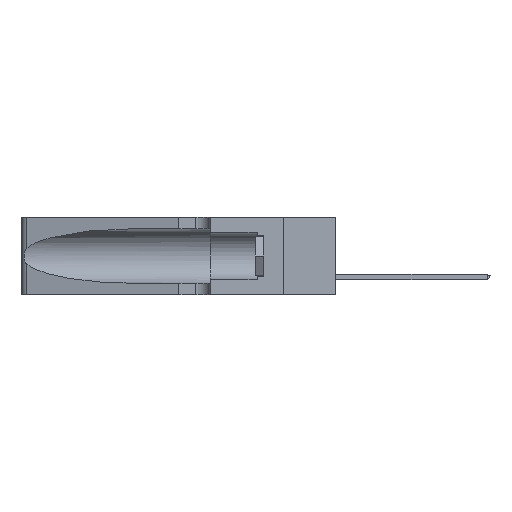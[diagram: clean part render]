
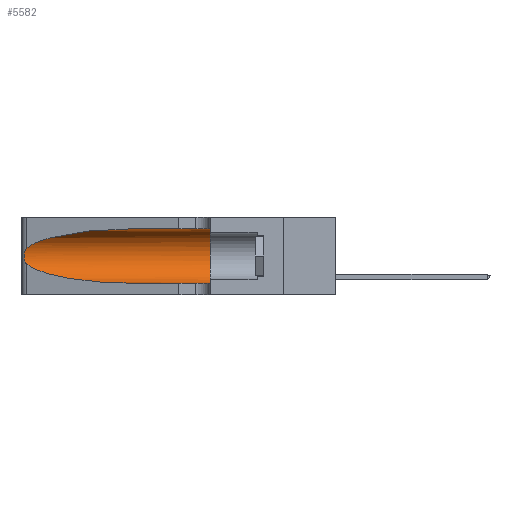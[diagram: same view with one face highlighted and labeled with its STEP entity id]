
A CAD part, left-side view. The second image highlights one B-rep face of the part: STEP entity #5582.
In plain terms, the highlighted cylindrical face has radius 3.308 mm (diameter 6.617 mm), a partial arc.
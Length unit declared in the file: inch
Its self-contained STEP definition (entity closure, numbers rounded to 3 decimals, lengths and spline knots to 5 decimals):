
#102 = CARTESIAN_POINT ( 'NONE',  ( 0.18966, 0.96281, 0.05475 ) ) ;
#1041 = CARTESIAN_POINT ( 'NONE',  ( 0.25787, 1.23484, 0.2124 ) ) ;
#1892 = CARTESIAN_POINT ( 'NONE',  ( 0.25555, 1.22994, 0.2215 ) ) ;
#1995 = CARTESIAN_POINT ( 'NONE',  ( 0.25856, 1.23593, 0.16098 ) ) ;
#2781 = DIRECTION ( 'NONE',  ( 0., -1., 0. ) ) ;
#3120 = CARTESIAN_POINT ( 'NONE',  ( 0.25487, 1.22718, 0.14631 ) ) ;
#3766 = CARTESIAN_POINT ( 'NONE',  ( 0.1305, 0.72297, 0.31525 ) ) ;
#3886 = CARTESIAN_POINT ( 'NONE',  ( 0.1305, 0.35, 0.31525 ) ) ;
#4468 = AXIS2_PLACEMENT_3D ( 'NONE', #6977, #22990, #28528 ) ;
#4597 = CARTESIAN_POINT ( 'NONE',  ( 0.1305, 0.72297, 0.05475 ) ) ;
#5565 = VERTEX_POINT ( 'NONE', #4597 ) ;
#5582 = ADVANCED_FACE ( 'NONE', ( #6471 ), #18770, .F. ) ;
#6172 = ORIENTED_EDGE ( 'NONE', *, *, #31013, .T. ) ;
#6341 = CARTESIAN_POINT ( 'NONE',  ( 0.25789, 1.23486, 0.15765 ) ) ;
#6422 = EDGE_CURVE ( 'NONE', #12882, #8485, #19596, .T. ) ;
#6471 = FACE_OUTER_BOUND ( 'NONE', #26349, .T. ) ;
#6977 = CARTESIAN_POINT ( 'NONE',  ( 0.1305, 0.35, 0.185 ) ) ;
#6988 = DIRECTION ( 'NONE',  ( 0., -1., 0. ) ) ;
#7961 = DIRECTION ( 'NONE',  ( 0., 0., -1. ) ) ;
#8222 = ORIENTED_EDGE ( 'NONE', *, *, #23806, .T. ) ;
#8485 = VERTEX_POINT ( 'NONE', #11077 ) ;
#8730 = VERTEX_POINT ( 'NONE', #3886 ) ;
#8903 = LINE ( 'NONE', #31170, #16921 ) ;
#10920 = CARTESIAN_POINT ( 'NONE',  ( 0.1305, 0.72297, 0.05475 ) ) ;
#11077 = CARTESIAN_POINT ( 'NONE',  ( 0.25487, 1.22718, 0.22369 ) ) ;
#12882 = VERTEX_POINT ( 'NONE', #3766 ) ;
#13686 = ORIENTED_EDGE ( 'NONE', *, *, #14118, .F. ) ;
#14118 = EDGE_CURVE ( 'NONE', #8730, #18132, #25139, .T. ) ;
#15327 = CARTESIAN_POINT ( 'NONE',  ( 0.1305, 0.35, 0.05475 ) ) ;
#15395 = CARTESIAN_POINT ( 'NONE',  ( 0.25639, 1.23184, 0.21858 ) ) ;
#15522 = CARTESIAN_POINT ( 'NONE',  ( 0.25487, 1.22718, 0.22369 ) ) ;
#16843 = VERTEX_POINT ( 'NONE', #3120 ) ;
#16921 = VECTOR ( 'NONE', #23068, 39.37008 ) ;
#17979 = CARTESIAN_POINT ( 'NONE',  ( 0.25854, 1.2359, 0.20912 ) ) ;
#18132 = VERTEX_POINT ( 'NONE', #15327 ) ;
#18770 = CYLINDRICAL_SURFACE ( 'NONE', #24945, 0.13025 ) ;
#18879 = CARTESIAN_POINT ( 'NONE',  ( 0.25487, 1.22718, 0.22369 ) ) ;
#19596 =( BOUNDED_CURVE ( )  B_SPLINE_CURVE ( 3, ( #24114, #31475, #32554, #18879 ),
 .UNSPECIFIED., .F., .F. ) 
 B_SPLINE_CURVE_WITH_KNOTS ( ( 4, 4 ),
 ( 1.5708, 2.84003 ),
 .UNSPECIFIED. ) 
 CURVE ( )  GEOMETRIC_REPRESENTATION_ITEM ( )  RATIONAL_B_SPLINE_CURVE ( ( 1., 0.87, 0.87, 1. ) ) 
 REPRESENTATION_ITEM ( '' )  );
#19973 = CARTESIAN_POINT ( 'NONE',  ( 0.25639, 1.23186, 0.15144 ) ) ;
#20278 = CARTESIAN_POINT ( 'NONE',  ( 0.1305, 1.61858, 0.31525 ) ) ;
#20600 = CARTESIAN_POINT ( 'NONE',  ( 0.26017, 1.23833, 0.17102 ) ) ;
#21375 = EDGE_CURVE ( 'NONE', #16843, #5565, #28964, .T. ) ;
#22990 = DIRECTION ( 'NONE',  ( 0., 1., 0. ) ) ;
#23068 = DIRECTION ( 'NONE',  ( 0., -1., 0. ) ) ;
#23806 = EDGE_CURVE ( 'NONE', #8485, #16843, #30666, .T. ) ;
#23840 = VECTOR ( 'NONE', #6988, 39.37008 ) ;
#24114 = CARTESIAN_POINT ( 'NONE',  ( 0.1305, 0.72297, 0.31525 ) ) ;
#24401 = CARTESIAN_POINT ( 'NONE',  ( 0.25487, 1.22718, 0.14631 ) ) ;
#24509 = CARTESIAN_POINT ( 'NONE',  ( 0.2373, 1.15595, 0.08982 ) ) ;
#24945 = AXIS2_PLACEMENT_3D ( 'NONE', #34987, #2781, #7961 ) ;
#25139 = CIRCLE ( 'NONE', #4468, 0.13025 ) ;
#26349 = EDGE_LOOP ( 'NONE', ( #27665, #8222, #26922, #6172, #13686, #34282 ) ) ;
#26922 = ORIENTED_EDGE ( 'NONE', *, *, #21375, .T. ) ;
#27665 = ORIENTED_EDGE ( 'NONE', *, *, #6422, .T. ) ;
#28025 = CARTESIAN_POINT ( 'NONE',  ( 0.26018, 1.23835, 0.19895 ) ) ;
#28528 = DIRECTION ( 'NONE',  ( 0., 0., 1. ) ) ;
#28964 =( BOUNDED_CURVE ( )  B_SPLINE_CURVE ( 3, ( #24401, #24509, #102, #10920 ),
 .UNSPECIFIED., .F., .F. ) 
 B_SPLINE_CURVE_WITH_KNOTS ( ( 4, 4 ),
 ( 3.44316, 4.71239 ),
 .UNSPECIFIED. ) 
 CURVE ( )  GEOMETRIC_REPRESENTATION_ITEM ( )  RATIONAL_B_SPLINE_CURVE ( ( 1., 0.87, 0.87, 1. ) ) 
 REPRESENTATION_ITEM ( '' )  );
#30666 = B_SPLINE_CURVE_WITH_KNOTS ( 'NONE', 3,
 ( #15522, #1892, #15395, #1041, #17979, #28025, #34258, #30832, #20600, #1995, #6341, #19973, #30718, #34025 ),
 .UNSPECIFIED., .F., .F.,
 ( 4, 2, 2, 2, 2, 2, 4 ),
 ( 0., 0.00027, 0.00053, 0.00107, 0.0016, 0.00187, 0.00214 ),
 .UNSPECIFIED. ) ;
#30718 = CARTESIAN_POINT ( 'NONE',  ( 0.25555, 1.22993, 0.14849 ) ) ;
#30832 = CARTESIAN_POINT ( 'NONE',  ( 0.26075, 1.23896, 0.178 ) ) ;
#30982 = LINE ( 'NONE', #20278, #23840 ) ;
#31013 = EDGE_CURVE ( 'NONE', #5565, #18132, #8903, .T. ) ;
#31170 = CARTESIAN_POINT ( 'NONE',  ( 0.1305, 1.61858, 0.05475 ) ) ;
#31475 = CARTESIAN_POINT ( 'NONE',  ( 0.18966, 0.96281, 0.31525 ) ) ;
#32554 = CARTESIAN_POINT ( 'NONE',  ( 0.2373, 1.15595, 0.28018 ) ) ;
#34025 = CARTESIAN_POINT ( 'NONE',  ( 0.25487, 1.22718, 0.14631 ) ) ;
#34258 = CARTESIAN_POINT ( 'NONE',  ( 0.26075, 1.23896, 0.19203 ) ) ;
#34282 = ORIENTED_EDGE ( 'NONE', *, *, #34842, .F. ) ;
#34842 = EDGE_CURVE ( 'NONE', #12882, #8730, #30982, .T. ) ;
#34987 = CARTESIAN_POINT ( 'NONE',  ( 0.1305, 1.61858, 0.185 ) ) ;
